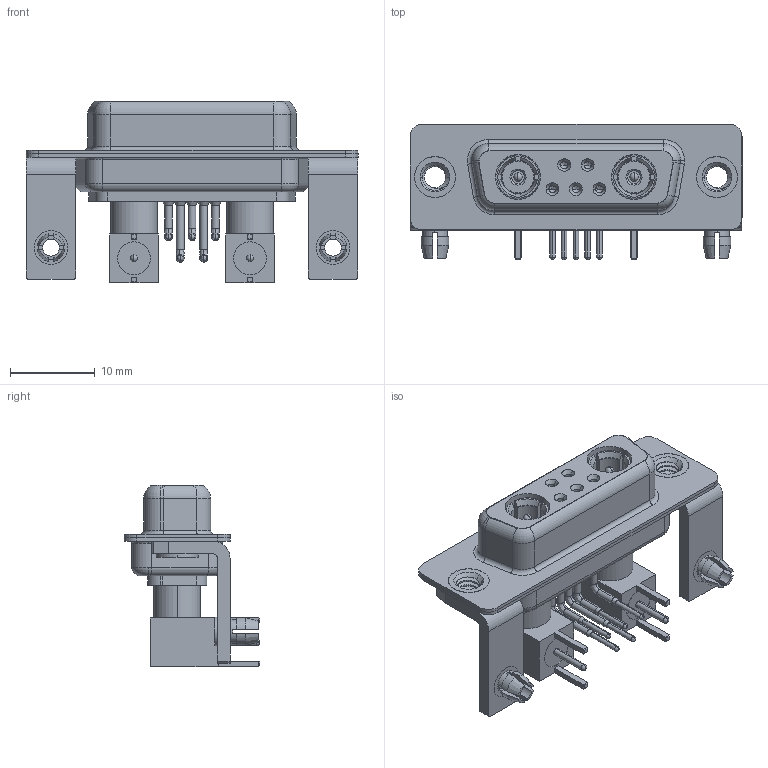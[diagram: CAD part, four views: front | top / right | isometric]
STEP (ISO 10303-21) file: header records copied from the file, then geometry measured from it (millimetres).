
FILE_DESCRIPTION (( 'STEP AP203' ), '1' );
FILE_NAME ('630-7W2-240-5TB.STEP', '2022-05-31T01:21:29', ( '' ), ( '' ), 'SwSTEP 2.0', 'SolidWorks 2020', '' );
FILE_SCHEMA (( 'CONFIG_CONTROL_DESIGN' ));
Length unit declared in the file: millimetre
Products named in the file (17): RA Back Shell; 630Combo Housing_7W2; Insulator Pin_Straight PC Tail; Insulator RA Pin; 630Combo Shell Front_15 Contacts; Co-Ax Plug Assy_RA; Pin_RA; 630Combo Threaded Rivet_B; Locking Collar; 630-7W2-240-5TB; 630Combo Stabilizer Bracket; 630Combo Shell Rear_15 Contacts; 630Combo Contact Row 2; 630Combo Board Lock; 630Combo Contact Row 1; Co-Ax Plug_RA PC Tail
Assembly tree (28 placements, depth 3):
  630-7W2-240-5TB
    630Combo Housing_7W2
    630Combo Shell Front_15 Contacts
    630Combo Shell Rear_15 Contacts
    630Combo Threaded Rivet_B  x2
    630Combo Stabilizer Bracket  x2
    630Combo Board Lock  x2
    Co-Ax Plug Assy_RA
      Co-Ax Plug_RA PC Tail
      Insulator Pin_Straight PC Tail
      Pin_RA
      Locking Collar
      RA Back Shell
      Insulator RA Pin
    Co-Ax Plug Assy_RA
      Co-Ax Plug_RA PC Tail
      Insulator Pin_Straight PC Tail
      Pin_RA
      Locking Collar
      RA Back Shell
      Insulator RA Pin
    630Combo Contact Row 1  x2
    630Combo Contact Row 2  x3
Bounding box: 39.2 x 16 x 21.41 mm (x, y, z)
Volume: 3271.3 mm3; surface area: 8124.1 mm2
Topology: 26 solids, 26 shells, 1010 faces, 2506 edges, 1580 vertices
Faces by surface type: cylinder 432, plane 344, cone 129, torus 69, bspline 28, sphere 8
Entity records: 22587 total; most frequent: CARTESIAN_POINT 5213, DIRECTION 3441, ORIENTED_EDGE 3046, EDGE_CURVE 1523, AXIS2_PLACEMENT_3D 1387, VERTEX_POINT 969, CIRCLE 737, EDGE_LOOP 718
